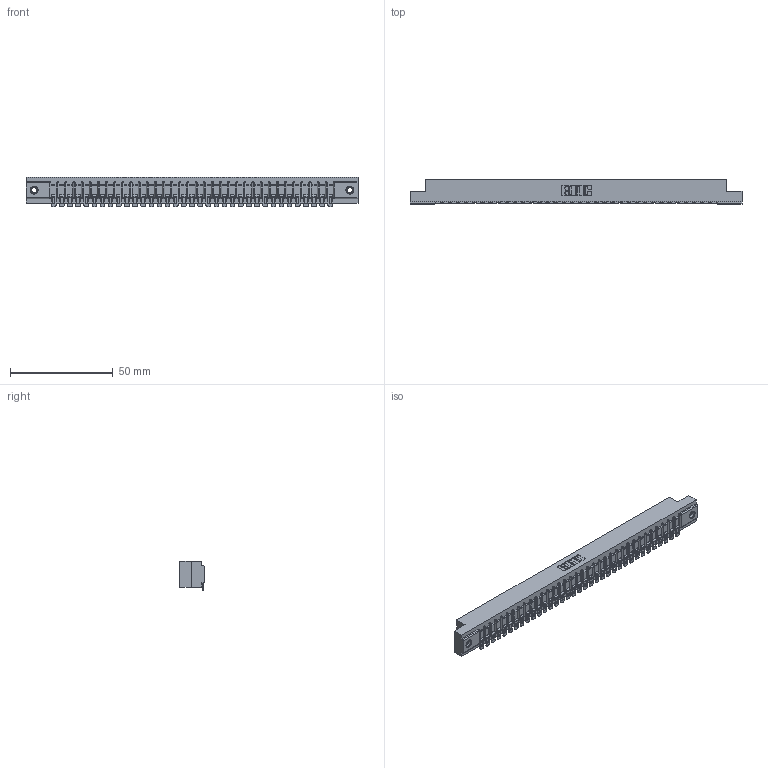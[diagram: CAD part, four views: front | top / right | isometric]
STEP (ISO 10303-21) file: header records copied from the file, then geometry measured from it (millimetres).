
FILE_DESCRIPTION (( 'STEP AP203' ), '1' );
FILE_NAME ('307-035-454-107.STEP', '2020-09-28T23:51:04', ( '' ), ( '' ), 'SwSTEP 2.0', 'SolidWorks 2020', '' );
FILE_SCHEMA (( 'CONFIG_CONTROL_DESIGN' ));
Length unit declared in the file: inch
Products named in the file (4): 345-250-001_345-250-005-103; 307-035-454-107; 307 Part_.156 Dia Mounting Holes; 307-290-002_554
Assembly tree (38 placements, depth 2):
  307-035-454-107
    307 Part_.156 Dia Mounting Holes
    307-290-002_554  x35
    345-250-001_345-250-005-103  x2
Bounding box: 161.7 x 12.01 x 14.52 mm (x, y, z)
Volume: 17250.5 mm3; surface area: 21704.1 mm2
Topology: 38 solids, 38 shells, 3049 faces, 9314 edges, 6104 vertices
Faces by surface type: plane 1712, cylinder 1249, sphere 72, cone 12, torus 4
Entity records: 33018 total; most frequent: CARTESIAN_POINT 5549, ORIENTED_EDGE 5532, DIRECTION 5410, EDGE_CURVE 2766, VECTOR 2108, LINE 2108, VERTEX_POINT 1790, AXIS2_PLACEMENT_3D 1651
